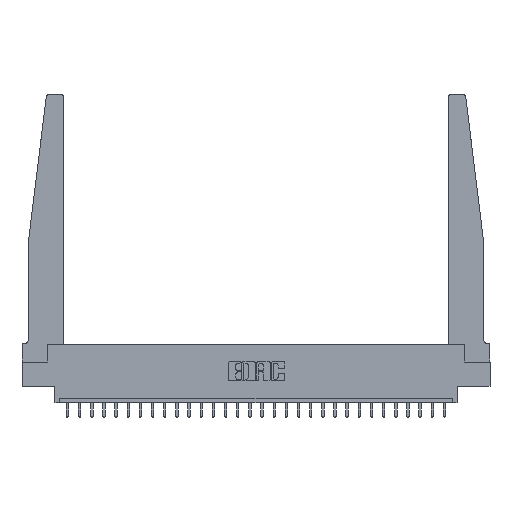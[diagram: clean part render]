
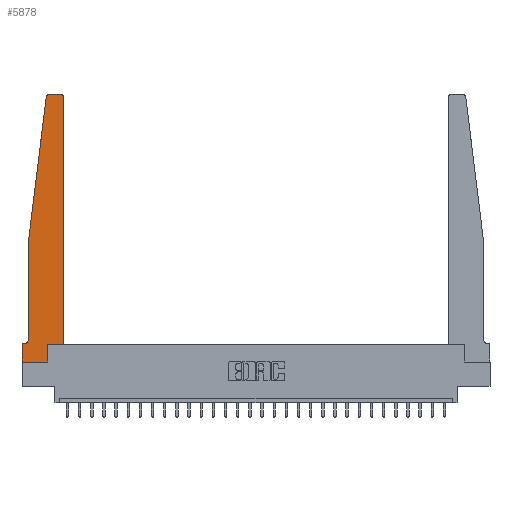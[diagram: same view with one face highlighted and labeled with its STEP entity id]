
A CAD part, top view. The second image highlights one B-rep face of the part: STEP entity #5878.
In plain terms, the highlighted planar face has unit normal (0, 0, 1).
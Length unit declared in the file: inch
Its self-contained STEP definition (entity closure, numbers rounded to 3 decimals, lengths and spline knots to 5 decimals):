
#647 = AXIS2_PLACEMENT_3D ( 'NONE', #9888, #21991, #5826 ) ;
#784 = VERTEX_POINT ( 'NONE', #2062 ) ;
#1169 = DIRECTION ( 'NONE',  ( -0.122, -0.992, 0. ) ) ;
#1170 = CARTESIAN_POINT ( 'NONE',  ( 0.24675, 2.72367, 0.37 ) ) ;
#1191 = DIRECTION ( 'NONE',  ( 0., -1., 0. ) ) ;
#1196 = DIRECTION ( 'NONE',  ( 0., 0., 1. ) ) ;
#1274 = CARTESIAN_POINT ( 'NONE',  ( 0.065, 1.25, 0.37 ) ) ;
#1438 = CARTESIAN_POINT ( 'NONE',  ( 0.065, 1.25, 0.37 ) ) ;
#1894 = DIRECTION ( 'NONE',  ( 0., 0., 1. ) ) ;
#2062 = CARTESIAN_POINT ( 'NONE',  ( 0.2605, 0., 0.37 ) ) ;
#2943 = AXIS2_PLACEMENT_3D ( 'NONE', #13995, #1894, #9704 ) ;
#3128 = ORIENTED_EDGE ( 'NONE', *, *, #12582, .T. ) ;
#3313 = CARTESIAN_POINT ( 'NONE',  ( 0.25, 2.75, 0.37 ) ) ;
#3452 = LINE ( 'NONE', #7614, #15453 ) ;
#3548 = VECTOR ( 'NONE', #1169, 39.37008 ) ;
#4210 = LINE ( 'NONE', #18861, #6862 ) ;
#4230 = CIRCLE ( 'NONE', #2943, 0.03 ) ;
#4704 = LINE ( 'NONE', #4962, #26369 ) ;
#4962 = CARTESIAN_POINT ( 'NONE',  ( 0.065, 1.25, 0.37 ) ) ;
#5096 = ORIENTED_EDGE ( 'NONE', *, *, #15572, .T. ) ;
#5643 = CARTESIAN_POINT ( 'NONE',  ( 0.2605, 0.18, 0.37 ) ) ;
#5826 = DIRECTION ( 'NONE',  ( 1., 0., 0. ) ) ;
#5878 = ADVANCED_FACE ( 'NONE', ( #19940 ), #23998, .T. ) ;
#6574 = CARTESIAN_POINT ( 'NONE',  ( 0.015, 0.2375, 0.37 ) ) ;
#6720 = CARTESIAN_POINT ( 'NONE',  ( 0.2605, 0.18, 0.37 ) ) ;
#6862 = VECTOR ( 'NONE', #8266, 39.37008 ) ;
#7366 = AXIS2_PLACEMENT_3D ( 'NONE', #7514, #1196, #15708 ) ;
#7514 = CARTESIAN_POINT ( 'NONE',  ( 0.27653, 2.72, 0.37 ) ) ;
#7565 = EDGE_CURVE ( 'NONE', #14642, #14032, #16665, .T. ) ;
#7614 = CARTESIAN_POINT ( 'NONE',  ( 0., 0., 0.37 ) ) ;
#7629 = EDGE_CURVE ( 'NONE', #784, #25732, #12773, .T. ) ;
#7769 = ORIENTED_EDGE ( 'NONE', *, *, #7629, .T. ) ;
#8067 = VERTEX_POINT ( 'NONE', #26095 ) ;
#8266 = DIRECTION ( 'NONE',  ( 0., 1., 0. ) ) ;
#8432 = VERTEX_POINT ( 'NONE', #13865 ) ;
#8492 = VECTOR ( 'NONE', #15877, 39.37008 ) ;
#8757 = DIRECTION ( 'NONE',  ( 0., 1., 0. ) ) ;
#9446 = CARTESIAN_POINT ( 'NONE',  ( 0., 0.1875, 0.37 ) ) ;
#9699 = LINE ( 'NONE', #20302, #8492 ) ;
#9704 = DIRECTION ( 'NONE',  ( 1., 0., 0. ) ) ;
#9723 = EDGE_CURVE ( 'NONE', #14032, #8067, #9699, .T. ) ;
#9888 = CARTESIAN_POINT ( 'NONE',  ( 0., 0.1875, 0.37 ) ) ;
#10997 = VERTEX_POINT ( 'NONE', #21281 ) ;
#11170 = EDGE_CURVE ( 'NONE', #10997, #16889, #4230, .T. ) ;
#11235 = CIRCLE ( 'NONE', #7366, 0.03 ) ;
#11628 = VECTOR ( 'NONE', #12401, 39.37008 ) ;
#11738 = CARTESIAN_POINT ( 'NONE',  ( 0.395, 2.75, 0.37 ) ) ;
#11843 = CARTESIAN_POINT ( 'NONE',  ( 0.27653, 2.75, 0.37 ) ) ;
#11901 = VECTOR ( 'NONE', #24870, 39.37008 ) ;
#12013 = EDGE_CURVE ( 'NONE', #8067, #784, #3452, .T. ) ;
#12316 = ORIENTED_EDGE ( 'NONE', *, *, #22842, .T. ) ;
#12401 = DIRECTION ( 'NONE',  ( 1., 0., 0. ) ) ;
#12582 = EDGE_CURVE ( 'NONE', #25732, #8432, #14692, .T. ) ;
#12773 = LINE ( 'NONE', #6720, #14469 ) ;
#12915 = CARTESIAN_POINT ( 'NONE',  ( 0.065, 0.1875, 0.37 ) ) ;
#13727 = VECTOR ( 'NONE', #17300, 39.37008 ) ;
#13865 = CARTESIAN_POINT ( 'NONE',  ( 0.425, 0.18, 0.37 ) ) ;
#13943 = VERTEX_POINT ( 'NONE', #11843 ) ;
#13995 = CARTESIAN_POINT ( 'NONE',  ( 0.395, 2.72, 0.37 ) ) ;
#14032 = VERTEX_POINT ( 'NONE', #9446 ) ;
#14089 = CARTESIAN_POINT ( 'NONE',  ( 0.015, 0.1875, 0.37 ) ) ;
#14288 = CARTESIAN_POINT ( 'NONE',  ( 0.425, 0.18, 0.37 ) ) ;
#14469 = VECTOR ( 'NONE', #8757, 39.37008 ) ;
#14642 = VERTEX_POINT ( 'NONE', #14089 ) ;
#14692 = LINE ( 'NONE', #14288, #11628 ) ;
#14773 = DIRECTION ( 'NONE',  ( -1., 0., 0. ) ) ;
#15209 = ORIENTED_EDGE ( 'NONE', *, *, #11170, .T. ) ;
#15453 = VECTOR ( 'NONE', #22133, 39.37008 ) ;
#15561 = LINE ( 'NONE', #3313, #13727 ) ;
#15572 = EDGE_CURVE ( 'NONE', #25356, #21785, #4704, .T. ) ;
#15708 = DIRECTION ( 'NONE',  ( 1., 0., 0. ) ) ;
#15877 = DIRECTION ( 'NONE',  ( 0., -1., 0. ) ) ;
#15994 = CIRCLE ( 'NONE', #18993, 0.05 ) ;
#16665 = LINE ( 'NONE', #12915, #11901 ) ;
#16889 = VERTEX_POINT ( 'NONE', #11738 ) ;
#16943 = ORIENTED_EDGE ( 'NONE', *, *, #7565, .T. ) ;
#17300 = DIRECTION ( 'NONE',  ( -1., 0., 0. ) ) ;
#17438 = ORIENTED_EDGE ( 'NONE', *, *, #26023, .T. ) ;
#17705 = LINE ( 'NONE', #1438, #3548 ) ;
#17988 = ORIENTED_EDGE ( 'NONE', *, *, #22230, .T. ) ;
#18457 = EDGE_LOOP ( 'NONE', ( #17988, #20325, #20702, #5096, #17438, #16943, #26348, #23427, #7769, #3128, #12316, #15209 ) ) ;
#18861 = CARTESIAN_POINT ( 'NONE',  ( 0.425, 0.18, 0.37 ) ) ;
#18993 = AXIS2_PLACEMENT_3D ( 'NONE', #6574, #19313, #14773 ) ;
#19098 = VERTEX_POINT ( 'NONE', #1170 ) ;
#19313 = DIRECTION ( 'NONE',  ( 0., 0., -1. ) ) ;
#19940 = FACE_OUTER_BOUND ( 'NONE', #18457, .T. ) ;
#20302 = CARTESIAN_POINT ( 'NONE',  ( 0., 0., 0.37 ) ) ;
#20325 = ORIENTED_EDGE ( 'NONE', *, *, #24466, .T. ) ;
#20702 = ORIENTED_EDGE ( 'NONE', *, *, #26205, .T. ) ;
#21281 = CARTESIAN_POINT ( 'NONE',  ( 0.425, 2.72, 0.37 ) ) ;
#21785 = VERTEX_POINT ( 'NONE', #23680 ) ;
#21991 = DIRECTION ( 'NONE',  ( 0., 0., 1. ) ) ;
#22133 = DIRECTION ( 'NONE',  ( 1., 0., 0. ) ) ;
#22230 = EDGE_CURVE ( 'NONE', #16889, #13943, #15561, .T. ) ;
#22842 = EDGE_CURVE ( 'NONE', #8432, #10997, #4210, .T. ) ;
#23427 = ORIENTED_EDGE ( 'NONE', *, *, #12013, .T. ) ;
#23680 = CARTESIAN_POINT ( 'NONE',  ( 0.065, 0.2375, 0.37 ) ) ;
#23998 = PLANE ( 'NONE',  #647 ) ;
#24466 = EDGE_CURVE ( 'NONE', #13943, #19098, #11235, .T. ) ;
#24870 = DIRECTION ( 'NONE',  ( -1., 0., 0. ) ) ;
#25356 = VERTEX_POINT ( 'NONE', #1274 ) ;
#25732 = VERTEX_POINT ( 'NONE', #5643 ) ;
#26023 = EDGE_CURVE ( 'NONE', #21785, #14642, #15994, .T. ) ;
#26095 = CARTESIAN_POINT ( 'NONE',  ( 0., 0., 0.37 ) ) ;
#26205 = EDGE_CURVE ( 'NONE', #19098, #25356, #17705, .T. ) ;
#26348 = ORIENTED_EDGE ( 'NONE', *, *, #9723, .T. ) ;
#26369 = VECTOR ( 'NONE', #1191, 39.37008 ) ;
